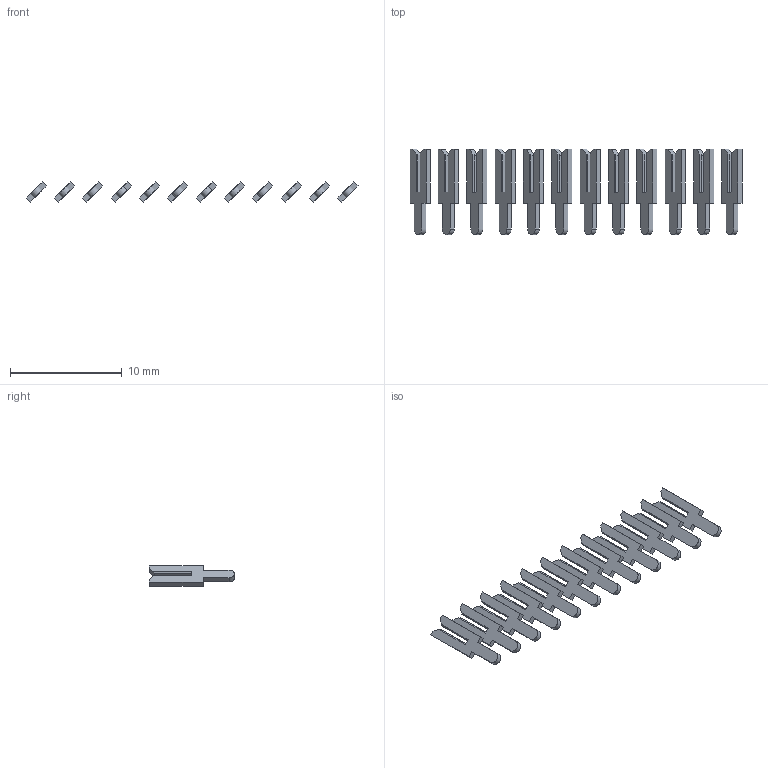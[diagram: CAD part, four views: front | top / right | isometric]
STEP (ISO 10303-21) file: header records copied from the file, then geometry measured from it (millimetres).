
FILE_DESCRIPTION (( 'STEP AP203' ), '1' );
FILE_NAME ('106-012-253-100.STEP', '2020-04-16T21:19:08', ( '' ), ( '' ), 'SwSTEP 2.0', 'SolidWorks 2016', '' );
FILE_SCHEMA (( 'CONFIG_CONTROL_DESIGN' ));
Length unit declared in the file: inch
Products named in the file (2): 100-290-001_100-290-253; 106-012-253-100
Assembly tree (12 placements, depth 2):
  106-012-253-100
    100-290-001_100-290-253  x12
Bounding box: 29.74 x 7.62 x 1.8 mm (x, y, z)
Volume: 66.2 mm3; surface area: 412.9 mm2
Topology: 12 solids, 12 shells, 240 faces, 648 edges, 432 vertices
Faces by surface type: plane 228, cylinder 12
Entity records: 1172 total; most frequent: DIRECTION 126, CARTESIAN_POINT 125, ORIENTED_EDGE 108, EDGE_CURVE 54, VECTOR 52, LINE 52, AXIS2_PLACEMENT_3D 37, VERTEX_POINT 36
